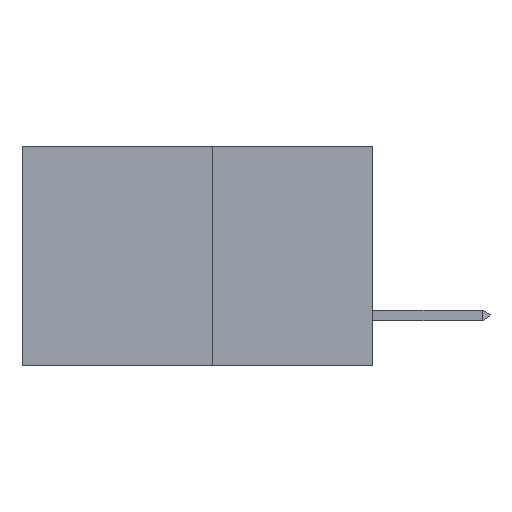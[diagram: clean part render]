
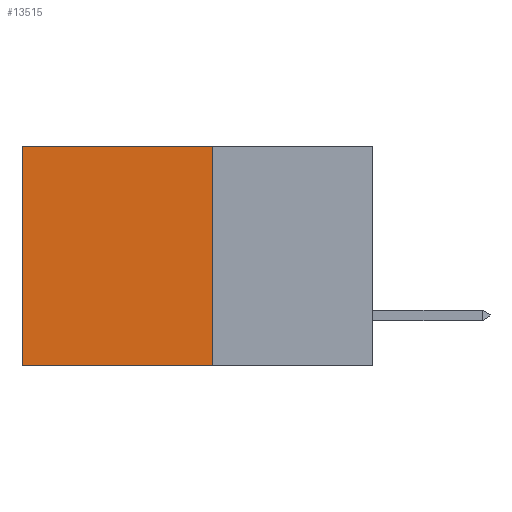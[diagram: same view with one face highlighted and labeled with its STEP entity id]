
A CAD part, left-side view. The second image highlights one B-rep face of the part: STEP entity #13515.
In plain terms, the highlighted planar face has unit normal (-1, 0, 0).
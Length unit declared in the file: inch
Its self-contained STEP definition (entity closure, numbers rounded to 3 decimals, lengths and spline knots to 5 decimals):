
#1048 = FACE_OUTER_BOUND ( 'NONE', #10360, .T. ) ;
#1056 = AXIS2_PLACEMENT_3D ( 'NONE', #2725, #3976, #12209 ) ;
#1124 = ORIENTED_EDGE ( 'NONE', *, *, #7054, .T. ) ;
#1488 = PLANE ( 'NONE',  #1056 ) ;
#2428 = VERTEX_POINT ( 'NONE', #6680 ) ;
#2518 = ORIENTED_EDGE ( 'NONE', *, *, #7654, .F. ) ;
#2725 = CARTESIAN_POINT ( 'NONE',  ( 0.277, 0.27, -0.37 ) ) ;
#3436 = DIRECTION ( 'NONE',  ( 0., 0., -1. ) ) ;
#3976 = DIRECTION ( 'NONE',  ( 1., 0., 0. ) ) ;
#4351 = VERTEX_POINT ( 'NONE', #14545 ) ;
#4353 = LINE ( 'NONE', #5692, #15273 ) ;
#5335 = LINE ( 'NONE', #8210, #11191 ) ;
#5603 = ORIENTED_EDGE ( 'NONE', *, *, #9259, .F. ) ;
#5692 = CARTESIAN_POINT ( 'NONE',  ( 0.277, 0.27, 0. ) ) ;
#6176 = VECTOR ( 'NONE', #11444, 39.37008 ) ;
#6680 = CARTESIAN_POINT ( 'NONE',  ( 0.277, 0.59, 0. ) ) ;
#7054 = EDGE_CURVE ( 'NONE', #2428, #14287, #11032, .T. ) ;
#7236 = DIRECTION ( 'NONE',  ( 0., 0., -1. ) ) ;
#7278 = LINE ( 'NONE', #10271, #6176 ) ;
#7654 = EDGE_CURVE ( 'NONE', #4351, #10442, #5335, .T. ) ;
#8210 = CARTESIAN_POINT ( 'NONE',  ( 0.277, 0.27, -0.37 ) ) ;
#8230 = EDGE_CURVE ( 'NONE', #4351, #2428, #4353, .T. ) ;
#9259 = EDGE_CURVE ( 'NONE', #10442, #14287, #7278, .T. ) ;
#10271 = CARTESIAN_POINT ( 'NONE',  ( 0.277, 0.27, -0.37 ) ) ;
#10360 = EDGE_LOOP ( 'NONE', ( #1124, #5603, #2518, #14821 ) ) ;
#10442 = VERTEX_POINT ( 'NONE', #13425 ) ;
#11032 = LINE ( 'NONE', #15299, #14094 ) ;
#11191 = VECTOR ( 'NONE', #3436, 39.37008 ) ;
#11444 = DIRECTION ( 'NONE',  ( 0., 1., 0. ) ) ;
#12209 = DIRECTION ( 'NONE',  ( 0., 0., -1. ) ) ;
#13425 = CARTESIAN_POINT ( 'NONE',  ( 0.277, 0.27, -0.37 ) ) ;
#13515 = ADVANCED_FACE ( 'NONE', ( #1048 ), #1488, .F. ) ;
#13823 = DIRECTION ( 'NONE',  ( 0., 1., 0. ) ) ;
#14094 = VECTOR ( 'NONE', #7236, 39.37008 ) ;
#14287 = VERTEX_POINT ( 'NONE', #14698 ) ;
#14545 = CARTESIAN_POINT ( 'NONE',  ( 0.277, 0.27, 0. ) ) ;
#14698 = CARTESIAN_POINT ( 'NONE',  ( 0.277, 0.59, -0.37 ) ) ;
#14821 = ORIENTED_EDGE ( 'NONE', *, *, #8230, .T. ) ;
#15273 = VECTOR ( 'NONE', #13823, 39.37008 ) ;
#15299 = CARTESIAN_POINT ( 'NONE',  ( 0.277, 0.59, -0.37 ) ) ;
